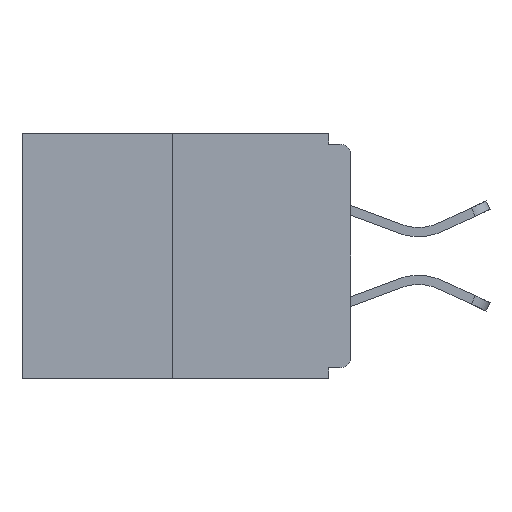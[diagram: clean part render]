
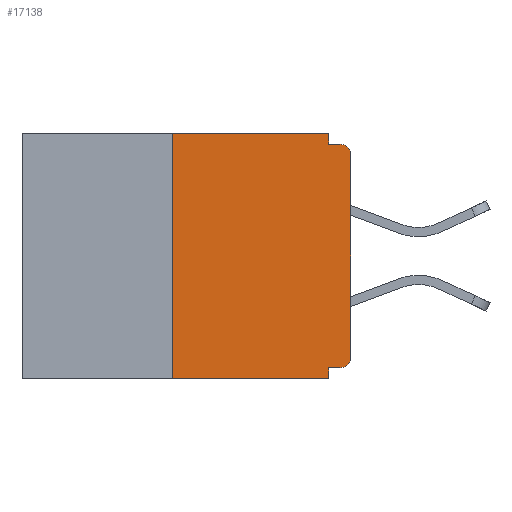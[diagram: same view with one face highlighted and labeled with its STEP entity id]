
A CAD part, left-side view. The second image highlights one B-rep face of the part: STEP entity #17138.
In plain terms, the highlighted planar face has unit normal (-1, 0, 0).
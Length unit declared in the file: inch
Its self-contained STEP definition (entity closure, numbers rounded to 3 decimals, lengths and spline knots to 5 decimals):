
#603 = ORIENTED_EDGE ( 'NONE', *, *, #16817, .F. ) ;
#690 = ORIENTED_EDGE ( 'NONE', *, *, #18009, .F. ) ;
#955 = CARTESIAN_POINT ( 'NONE',  ( 0., 0., 0. ) ) ;
#1056 = EDGE_CURVE ( 'NONE', #12142, #17153, #8984, .T. ) ;
#1178 = VECTOR ( 'NONE', #6835, 39.37008 ) ;
#1212 = CARTESIAN_POINT ( 'NONE',  ( 0., 0., -0.03 ) ) ;
#1569 = LINE ( 'NONE', #6266, #16274 ) ;
#1586 = CARTESIAN_POINT ( 'NONE',  ( 0., 0., -0.313 ) ) ;
#1943 = LINE ( 'NONE', #7642, #12985 ) ;
#2290 = DIRECTION ( 'NONE',  ( -1., 0., 0. ) ) ;
#2584 = CARTESIAN_POINT ( 'NONE',  ( 0., 0.25, 0. ) ) ;
#3087 = VERTEX_POINT ( 'NONE', #10826 ) ;
#3193 = VERTEX_POINT ( 'NONE', #12272 ) ;
#3233 = ORIENTED_EDGE ( 'NONE', *, *, #14525, .T. ) ;
#3236 = AXIS2_PLACEMENT_3D ( 'NONE', #4008, #12550, #6710 ) ;
#3389 = EDGE_CURVE ( 'NONE', #16557, #3087, #18752, .T. ) ;
#3432 = CARTESIAN_POINT ( 'NONE',  ( 0., 0.46, 0. ) ) ;
#3468 = VERTEX_POINT ( 'NONE', #17052 ) ;
#3695 = DIRECTION ( 'NONE',  ( 0., 0., -1. ) ) ;
#3705 = CARTESIAN_POINT ( 'NONE',  ( 0., 0.031, 0. ) ) ;
#4008 = CARTESIAN_POINT ( 'NONE',  ( 0., 0.46, 0. ) ) ;
#4478 = LINE ( 'NONE', #8475, #14352 ) ;
#4968 = ORIENTED_EDGE ( 'NONE', *, *, #7499, .F. ) ;
#5057 = CARTESIAN_POINT ( 'NONE',  ( 0., 0.015, -0.313 ) ) ;
#5631 = CARTESIAN_POINT ( 'NONE',  ( 0., 0.015, -0.328 ) ) ;
#5932 = EDGE_CURVE ( 'NONE', #3193, #3087, #4478, .T. ) ;
#6111 = CIRCLE ( 'NONE', #13462, 0.015 ) ;
#6266 = CARTESIAN_POINT ( 'NONE',  ( 0., 0.25, 0. ) ) ;
#6710 = DIRECTION ( 'NONE',  ( 0., 0., -1. ) ) ;
#6754 = VECTOR ( 'NONE', #16503, 39.37008 ) ;
#6835 = DIRECTION ( 'NONE',  ( 0., 0., 1. ) ) ;
#7214 = VECTOR ( 'NONE', #10554, 39.37008 ) ;
#7484 = VECTOR ( 'NONE', #18959, 39.37008 ) ;
#7499 = EDGE_CURVE ( 'NONE', #13363, #16557, #1943, .T. ) ;
#7642 = CARTESIAN_POINT ( 'NONE',  ( 0., 0., -0.328 ) ) ;
#7852 = CARTESIAN_POINT ( 'NONE',  ( 0., 0.031, 0. ) ) ;
#8051 = CIRCLE ( 'NONE', #12151, 0.015 ) ;
#8312 = DIRECTION ( 'NONE',  ( 0., 0., -1. ) ) ;
#8325 = ORIENTED_EDGE ( 'NONE', *, *, #17833, .F. ) ;
#8475 = CARTESIAN_POINT ( 'NONE',  ( 0., 0.46, -0.343 ) ) ;
#8984 = LINE ( 'NONE', #955, #1178 ) ;
#9427 = DIRECTION ( 'NONE',  ( 0., 0., -1. ) ) ;
#9434 = VERTEX_POINT ( 'NONE', #18156 ) ;
#9483 = EDGE_LOOP ( 'NONE', ( #8325, #15105, #12623, #17433, #4968, #11638, #14888, #3233, #603, #690 ) ) ;
#9950 = LINE ( 'NONE', #7852, #6754 ) ;
#10554 = DIRECTION ( 'NONE',  ( 0., -1., 0. ) ) ;
#10781 = EDGE_CURVE ( 'NONE', #3193, #13938, #1569, .T. ) ;
#10826 = CARTESIAN_POINT ( 'NONE',  ( 0., 0.031, -0.343 ) ) ;
#11638 = ORIENTED_EDGE ( 'NONE', *, *, #17030, .T. ) ;
#12003 = DIRECTION ( 'NONE',  ( 0., -1., 0. ) ) ;
#12142 = VERTEX_POINT ( 'NONE', #1586 ) ;
#12151 = AXIS2_PLACEMENT_3D ( 'NONE', #17101, #2290, #8312 ) ;
#12272 = CARTESIAN_POINT ( 'NONE',  ( 0., 0.25, -0.343 ) ) ;
#12482 = DIRECTION ( 'NONE',  ( -1., 0., 0. ) ) ;
#12550 = DIRECTION ( 'NONE',  ( 1., 0., 0. ) ) ;
#12623 = ORIENTED_EDGE ( 'NONE', *, *, #5932, .T. ) ;
#12725 = PLANE ( 'NONE',  #3236 ) ;
#12985 = VECTOR ( 'NONE', #13357, 39.37008 ) ;
#13357 = DIRECTION ( 'NONE',  ( 0., 1., 0. ) ) ;
#13363 = VERTEX_POINT ( 'NONE', #5631 ) ;
#13462 = AXIS2_PLACEMENT_3D ( 'NONE', #5057, #12482, #3695 ) ;
#13652 = LINE ( 'NONE', #3432, #7214 ) ;
#13726 = DIRECTION ( 'NONE',  ( 0., 0., 1. ) ) ;
#13938 = VERTEX_POINT ( 'NONE', #2584 ) ;
#14352 = VECTOR ( 'NONE', #12003, 39.37008 ) ;
#14382 = LINE ( 'NONE', #19020, #7484 ) ;
#14525 = EDGE_CURVE ( 'NONE', #17153, #3468, #8051, .T. ) ;
#14878 = VECTOR ( 'NONE', #9427, 39.37008 ) ;
#14888 = ORIENTED_EDGE ( 'NONE', *, *, #1056, .T. ) ;
#15105 = ORIENTED_EDGE ( 'NONE', *, *, #10781, .F. ) ;
#15473 = VERTEX_POINT ( 'NONE', #3705 ) ;
#16274 = VECTOR ( 'NONE', #13726, 39.37008 ) ;
#16503 = DIRECTION ( 'NONE',  ( 0., 0., -1. ) ) ;
#16557 = VERTEX_POINT ( 'NONE', #16850 ) ;
#16817 = EDGE_CURVE ( 'NONE', #9434, #3468, #14382, .T. ) ;
#16850 = CARTESIAN_POINT ( 'NONE',  ( 0., 0.031, -0.328 ) ) ;
#17030 = EDGE_CURVE ( 'NONE', #13363, #12142, #6111, .T. ) ;
#17052 = CARTESIAN_POINT ( 'NONE',  ( 0., 0.015, -0.015 ) ) ;
#17101 = CARTESIAN_POINT ( 'NONE',  ( 0., 0.015, -0.03 ) ) ;
#17138 = ADVANCED_FACE ( 'NONE', ( #18224 ), #12725, .F. ) ;
#17153 = VERTEX_POINT ( 'NONE', #1212 ) ;
#17433 = ORIENTED_EDGE ( 'NONE', *, *, #3389, .F. ) ;
#17833 = EDGE_CURVE ( 'NONE', #13938, #15473, #13652, .T. ) ;
#18009 = EDGE_CURVE ( 'NONE', #15473, #9434, #9950, .T. ) ;
#18156 = CARTESIAN_POINT ( 'NONE',  ( 0., 0.031, -0.015 ) ) ;
#18205 = CARTESIAN_POINT ( 'NONE',  ( 0., 0.031, -0.343 ) ) ;
#18224 = FACE_OUTER_BOUND ( 'NONE', #9483, .T. ) ;
#18752 = LINE ( 'NONE', #18205, #14878 ) ;
#18959 = DIRECTION ( 'NONE',  ( 0., -1., 0. ) ) ;
#19020 = CARTESIAN_POINT ( 'NONE',  ( 0., 0., -0.015 ) ) ;
